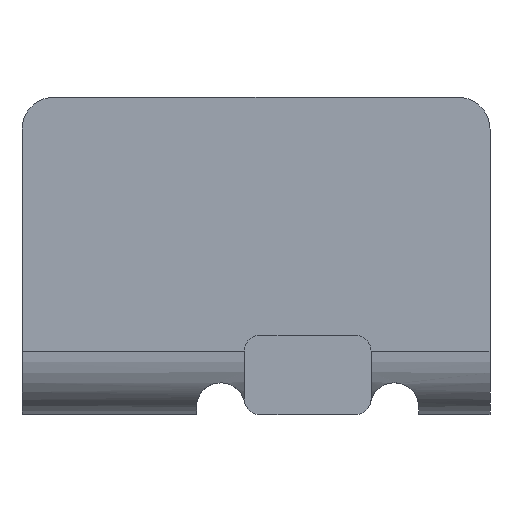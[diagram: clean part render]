
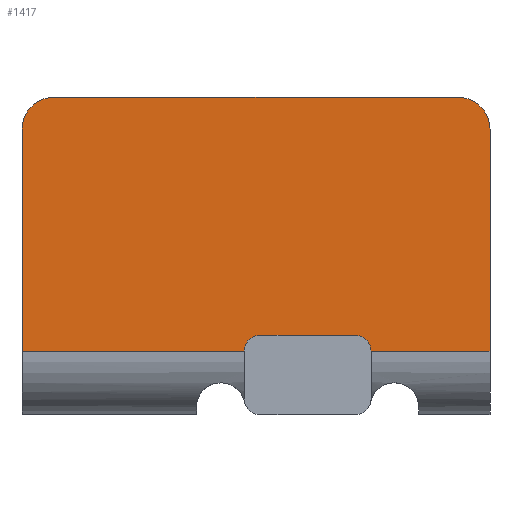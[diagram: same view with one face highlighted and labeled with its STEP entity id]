
A CAD part, left-side view. The second image highlights one B-rep face of the part: STEP entity #1417.
In plain terms, the highlighted planar face has unit normal (-1, 0, 0).
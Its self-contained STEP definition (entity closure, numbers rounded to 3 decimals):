
#252=CARTESIAN_POINT('',(-18.5,6.,-1.));
#253=VERTEX_POINT('',#252);
#470=CARTESIAN_POINT('',(-18.5,-2.0,-1.));
#471=VERTEX_POINT('',#470);
#920=CARTESIAN_POINT('',(-18.5,-9.5,13.0));
#921=VERTEX_POINT('',#920);
#928=CARTESIAN_POINT('',(-18.5,-9.5,-1.));
#929=VERTEX_POINT('',#928);
#930=CARTESIAN_POINT('',(-18.5,-9.5,-1.));
#931=DIRECTION('',(0.0,0.0,1.0));
#932=VECTOR('',#931,14.);
#933=LINE('',#930,#932);
#934=EDGE_CURVE('',#929,#921,#933,.T.);
#1103=CARTESIAN_POINT('',(-18.5,20.0,-1.));
#1104=VERTEX_POINT('',#1103);
#1112=CARTESIAN_POINT('',(-18.5,20.0,13.0));
#1113=VERTEX_POINT('',#1112);
#1114=CARTESIAN_POINT('',(-18.5,20.0,13.0));
#1115=DIRECTION('',(0.0,0.0,-1.0));
#1116=VECTOR('',#1115,14.);
#1117=LINE('',#1114,#1116);
#1118=EDGE_CURVE('',#1113,#1104,#1117,.T.);
#1219=CARTESIAN_POINT('',(-18.5,-1.0,0.0));
#1220=VERTEX_POINT('',#1219);
#1221=CARTESIAN_POINT('',(-18.5,-1.0,-1.0));
#1222=DIRECTION('',(1.0,0.0,0.0));
#1223=DIRECTION('',(0.0,-0.707,0.707));
#1224=AXIS2_PLACEMENT_3D('',#1221,#1222,#1223);
#1225=CIRCLE('',#1224,1.0);
#1226=EDGE_CURVE('',#471,#1220,#1225,.F.);
#1284=CARTESIAN_POINT('',(-18.5,5.,0.0));
#1285=VERTEX_POINT('',#1284);
#1292=CARTESIAN_POINT('',(-18.5,5.,-1.0));
#1293=DIRECTION('',(1.0,0.0,0.0));
#1294=DIRECTION('',(0.0,0.707,0.707));
#1295=AXIS2_PLACEMENT_3D('',#1292,#1293,#1294);
#1296=CIRCLE('',#1295,1.0);
#1297=EDGE_CURVE('',#1285,#253,#1296,.F.);
#1353=CARTESIAN_POINT('',(-18.5,-9.5,-1.));
#1354=DIRECTION('',(0.0,1.0,0.0));
#1355=VECTOR('',#1354,7.5);
#1356=LINE('',#1353,#1355);
#1357=EDGE_CURVE('',#929,#471,#1356,.T.);
#1369=CARTESIAN_POINT('',(-18.5,0.0,15.0));
#1370=DIRECTION('',(-1.0,0.0,0.0));
#1371=DIRECTION('',(0.0,0.0,1.0));
#1372=AXIS2_PLACEMENT_3D('',#1369,#1370,#1371);
#1373=PLANE('',#1372);
#1374=ORIENTED_EDGE('',*,*,#1357,.F.);
#1375=ORIENTED_EDGE('',*,*,#934,.T.);
#1376=CARTESIAN_POINT('',(-18.5,-7.5,15.0));
#1377=VERTEX_POINT('',#1376);
#1378=CARTESIAN_POINT('',(-18.5,-7.5,13.0));
#1379=DIRECTION('',(1.0,0.0,0.0));
#1380=DIRECTION('',(0.0,-0.707,0.707));
#1381=AXIS2_PLACEMENT_3D('',#1378,#1379,#1380);
#1382=CIRCLE('',#1381,2.0);
#1383=EDGE_CURVE('',#1377,#921,#1382,.T.);
#1384=ORIENTED_EDGE('',*,*,#1383,.F.);
#1385=CARTESIAN_POINT('',(-18.5,18.0,15.0));
#1386=VERTEX_POINT('',#1385);
#1387=CARTESIAN_POINT('',(-18.5,-7.5,15.0));
#1388=DIRECTION('',(0.0,1.0,0.0));
#1389=VECTOR('',#1388,25.5);
#1390=LINE('',#1387,#1389);
#1391=EDGE_CURVE('',#1377,#1386,#1390,.T.);
#1392=ORIENTED_EDGE('',*,*,#1391,.T.);
#1393=CARTESIAN_POINT('',(-18.5,18.0,13.0));
#1394=DIRECTION('',(1.0,0.0,0.0));
#1395=DIRECTION('',(0.0,0.707,0.707));
#1396=AXIS2_PLACEMENT_3D('',#1393,#1394,#1395);
#1397=CIRCLE('',#1396,2.0);
#1398=EDGE_CURVE('',#1113,#1386,#1397,.T.);
#1399=ORIENTED_EDGE('',*,*,#1398,.F.);
#1400=ORIENTED_EDGE('',*,*,#1118,.T.);
#1401=CARTESIAN_POINT('',(-18.5,6.,-1.));
#1402=DIRECTION('',(0.0,1.0,0.0));
#1403=VECTOR('',#1402,14.0);
#1404=LINE('',#1401,#1403);
#1405=EDGE_CURVE('',#253,#1104,#1404,.T.);
#1406=ORIENTED_EDGE('',*,*,#1405,.F.);
#1407=ORIENTED_EDGE('',*,*,#1297,.F.);
#1408=CARTESIAN_POINT('',(-18.5,5.,0.0));
#1409=DIRECTION('',(0.0,-1.0,0.0));
#1410=VECTOR('',#1409,6.);
#1411=LINE('',#1408,#1410);
#1412=EDGE_CURVE('',#1285,#1220,#1411,.T.);
#1413=ORIENTED_EDGE('',*,*,#1412,.T.);
#1414=ORIENTED_EDGE('',*,*,#1226,.F.);
#1415=EDGE_LOOP('',(#1374,#1375,#1384,#1392,#1399,#1400,#1406,#1407,#1413,#1414));
#1416=FACE_OUTER_BOUND('',#1415,.T.);
#1417=ADVANCED_FACE('',(#1416),#1373,.T.);
